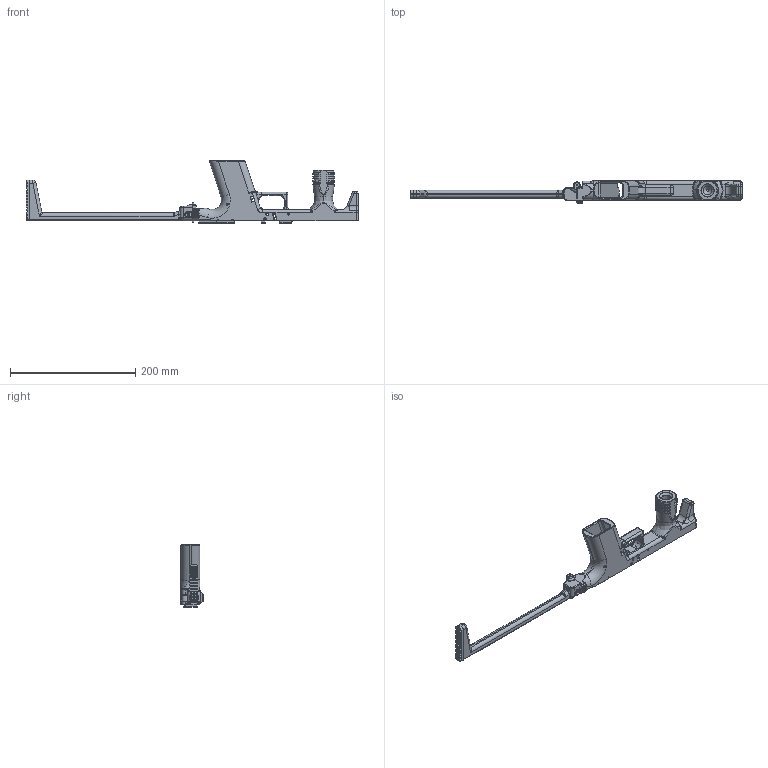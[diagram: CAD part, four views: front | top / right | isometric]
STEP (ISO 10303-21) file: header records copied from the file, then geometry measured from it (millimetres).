
FILE_DESCRIPTION(/* description */ (''),/* implementation_level */ '2;1');
FILE_NAME(/* name */ 'p80 PDW.stp',/* time_stamp */ '2019-12-27T01:01:52+02:00',/* author */ (''),/* organization */ (''),/* preprocessor_version */ 'ST-DEVELOPER v15.2',/* originating_system */ 'Autodesk Translator Framework v2.0.0.5431',/* authorisation */ '');
FILE_SCHEMA (('AUTOMOTIVE_DESIGN { 1 0 10303 214 3 1 1 }'));
Length unit declared in the file: centimetre
Products named in the file (1): GLOCK PDW V4 WORKING VERSION
Bounding box: 530.63 x 35.68 x 99.71 mm (x, y, z)
Volume: 258835.8 mm3; surface area: 120277 mm2
Topology: 12 solids, 12 shells, 1643 faces, 4257 edges, 2574 vertices
Faces by surface type: plane 602, cylinder 492, bspline 317, torus 119, cone 67, sphere 46
Full cylindrical faces by diameter (mm): 1.25 x8, 1.655 x8, 1.8 x1, 2.5 x5, 3.057 x4, 3.06 x3, 4 x3, 4.042 x2, 6.5 x1, 7.2 x1, 7.4 x1, 8 x1, 9 x1, 14 x1
Entity records: 58215 total; most frequent: CARTESIAN_POINT 20002, ORIENTED_EDGE 8230, DIRECTION 7540, EDGE_CURVE 4115, AXIS2_PLACEMENT_3D 2756, VERTEX_POINT 2552, LINE 2028, VECTOR 2028
